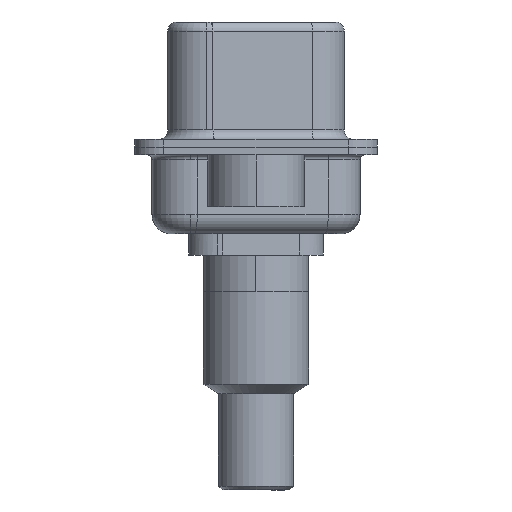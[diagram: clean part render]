
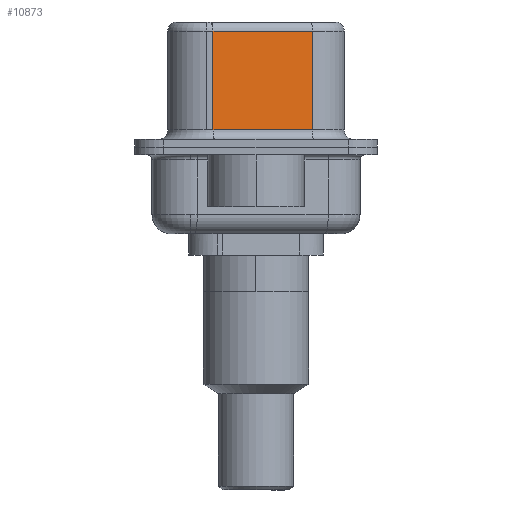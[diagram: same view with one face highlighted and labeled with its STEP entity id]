
A CAD part, left-side view. The second image highlights one B-rep face of the part: STEP entity #10873.
In plain terms, the highlighted planar face has unit normal (-0.985, -0.174, 0).
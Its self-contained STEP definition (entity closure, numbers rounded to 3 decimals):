
#90 = VERTEX_POINT ( 'NONE', #15751 ) ;
#506 = ORIENTED_EDGE ( 'NONE', *, *, #14365, .T. ) ;
#601 = ORIENTED_EDGE ( 'NONE', *, *, #1177, .T. ) ;
#810 = EDGE_CURVE ( 'NONE', #90, #6442, #21774, .T. ) ;
#1177 = EDGE_CURVE ( 'NONE', #14115, #9804, #22653, .T. ) ;
#1307 = ORIENTED_EDGE ( 'NONE', *, *, #810, .F. ) ;
#2900 = DIRECTION ( 'NONE',  ( 0.174, -0.985, 0. ) ) ;
#3718 = DIRECTION ( 'NONE',  ( 0., 0., -1. ) ) ;
#3922 = CARTESIAN_POINT ( 'NONE',  ( 4.58, -2.927, 6.52 ) ) ;
#5124 = DIRECTION ( 'NONE',  ( 0., 0., -1. ) ) ;
#5909 = DIRECTION ( 'NONE',  ( -0.174, 0.985, 0. ) ) ;
#6442 = VERTEX_POINT ( 'NONE', #12050 ) ;
#9792 = EDGE_CURVE ( 'NONE', #90, #14115, #11396, .T. ) ;
#9804 = VERTEX_POINT ( 'NONE', #16729 ) ;
#10873 = ADVANCED_FACE ( 'NONE', ( #21063 ), #11659, .F. ) ;
#11396 = LINE ( 'NONE', #19990, #15937 ) ;
#11659 = PLANE ( 'NONE',  #14746 ) ;
#12050 = CARTESIAN_POINT ( 'NONE',  ( 4.58, -2.927, 0.9 ) ) ;
#12390 = VECTOR ( 'NONE', #3718, 1000. ) ;
#13474 = LINE ( 'NONE', #14521, #23799 ) ;
#14115 = VERTEX_POINT ( 'NONE', #19603 ) ;
#14365 = EDGE_CURVE ( 'NONE', #9804, #6442, #13474, .T. ) ;
#14521 = CARTESIAN_POINT ( 'NONE',  ( 4.58, -2.927, 0.9 ) ) ;
#14746 = AXIS2_PLACEMENT_3D ( 'NONE', #3922, #17457, #5909 ) ;
#15751 = CARTESIAN_POINT ( 'NONE',  ( 4.58, -2.927, 6.02 ) ) ;
#15937 = VECTOR ( 'NONE', #20469, 1000. ) ;
#16576 = VECTOR ( 'NONE', #5124, 1000. ) ;
#16729 = CARTESIAN_POINT ( 'NONE',  ( 3.67, 2.233, 0.9 ) ) ;
#17457 = DIRECTION ( 'NONE',  ( 0.985, 0.174, 0. ) ) ;
#19603 = CARTESIAN_POINT ( 'NONE',  ( 3.67, 2.233, 6.02 ) ) ;
#19990 = CARTESIAN_POINT ( 'NONE',  ( 4.58, -2.927, 6.02 ) ) ;
#20469 = DIRECTION ( 'NONE',  ( -0.174, 0.985, 0. ) ) ;
#21063 = FACE_OUTER_BOUND ( 'NONE', #25181, .T. ) ;
#21774 = LINE ( 'NONE', #23072, #16576 ) ;
#22653 = LINE ( 'NONE', #24635, #12390 ) ;
#23072 = CARTESIAN_POINT ( 'NONE',  ( 4.58, -2.927, 6.52 ) ) ;
#23799 = VECTOR ( 'NONE', #2900, 1000. ) ;
#24635 = CARTESIAN_POINT ( 'NONE',  ( 3.67, 2.233, 6.52 ) ) ;
#24696 = ORIENTED_EDGE ( 'NONE', *, *, #9792, .T. ) ;
#25181 = EDGE_LOOP ( 'NONE', ( #1307, #24696, #601, #506 ) ) ;
